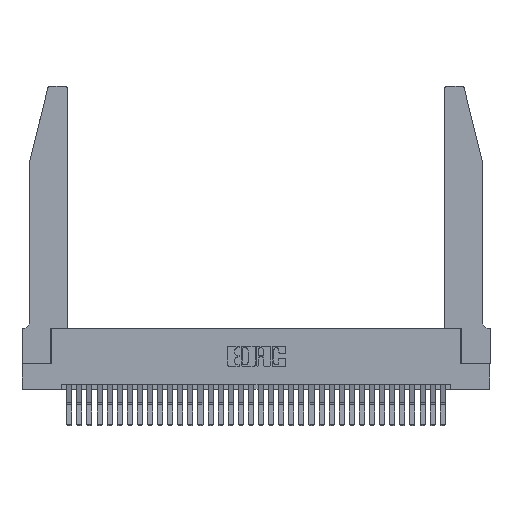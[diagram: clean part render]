
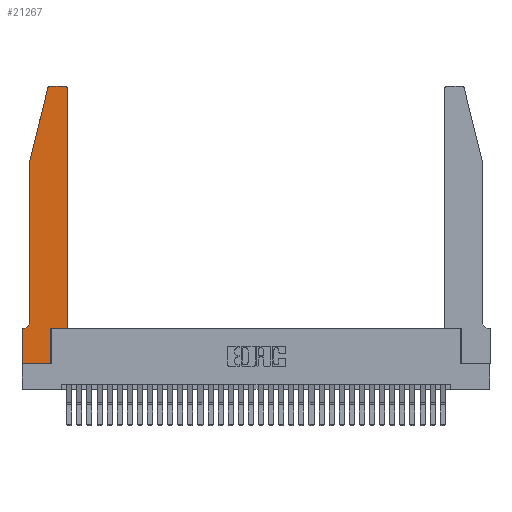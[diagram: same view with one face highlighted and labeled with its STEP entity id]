
A CAD part, top view. The second image highlights one B-rep face of the part: STEP entity #21267.
In plain terms, the highlighted planar face has unit normal (0, 0, 1).
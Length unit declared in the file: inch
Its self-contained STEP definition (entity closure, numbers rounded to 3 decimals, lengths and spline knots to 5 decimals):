
#935 = DIRECTION ( 'NONE',  ( 0., -1., 0. ) ) ;
#1201 = ORIENTED_EDGE ( 'NONE', *, *, #31372, .T. ) ;
#1291 = CARTESIAN_POINT ( 'NONE',  ( 0.0755, 2., 0.37 ) ) ;
#1376 = ORIENTED_EDGE ( 'NONE', *, *, #2684, .T. ) ;
#1956 = DIRECTION ( 'NONE',  ( 1., 0., 0. ) ) ;
#2573 = LINE ( 'NONE', #11858, #15707 ) ;
#2684 = EDGE_CURVE ( 'NONE', #17041, #10443, #32523, .T. ) ;
#2877 = CARTESIAN_POINT ( 'NONE',  ( 0., 0., 0.37 ) ) ;
#3199 = VECTOR ( 'NONE', #15643, 39.37008 ) ;
#3333 = LINE ( 'NONE', #8171, #29338 ) ;
#3379 = CARTESIAN_POINT ( 'NONE',  ( 0.0755, 0.35, 0.37 ) ) ;
#3596 = LINE ( 'NONE', #31079, #3199 ) ;
#3832 = ORIENTED_EDGE ( 'NONE', *, *, #15936, .T. ) ;
#4374 = DIRECTION ( 'NONE',  ( 0., 1., 0. ) ) ;
#4702 = CARTESIAN_POINT ( 'NONE',  ( 0.2865, 0.35, 0.37 ) ) ;
#5097 = VERTEX_POINT ( 'NONE', #31249 ) ;
#5255 = CARTESIAN_POINT ( 'NONE',  ( 0.0755, 2., 0.37 ) ) ;
#5286 = DIRECTION ( 'NONE',  ( 1., 0., 0. ) ) ;
#6070 = ORIENTED_EDGE ( 'NONE', *, *, #16744, .T. ) ;
#6346 = VERTEX_POINT ( 'NONE', #7007 ) ;
#6767 = EDGE_CURVE ( 'NONE', #12566, #17512, #3596, .T. ) ;
#7007 = CARTESIAN_POINT ( 'NONE',  ( 0.4505, 2.72, 0.37 ) ) ;
#7131 = AXIS2_PLACEMENT_3D ( 'NONE', #7559, #13362, #5286 ) ;
#7261 = AXIS2_PLACEMENT_3D ( 'NONE', #22783, #31485, #20400 ) ;
#7324 = PLANE ( 'NONE',  #7261 ) ;
#7491 = FACE_OUTER_BOUND ( 'NONE', #23174, .T. ) ;
#7559 = CARTESIAN_POINT ( 'NONE',  ( 0.4205, 2.72, 0.37 ) ) ;
#7577 = LINE ( 'NONE', #17139, #25419 ) ;
#7645 = CARTESIAN_POINT ( 'NONE',  ( 0.284, 2.72, 0.37 ) ) ;
#7892 = ORIENTED_EDGE ( 'NONE', *, *, #26715, .T. ) ;
#8171 = CARTESIAN_POINT ( 'NONE',  ( 0., 0., 0.37 ) ) ;
#8234 = CARTESIAN_POINT ( 'NONE',  ( 0., 0., 0.37 ) ) ;
#8263 = CARTESIAN_POINT ( 'NONE',  ( 0.0755, 0.42, 0.37 ) ) ;
#8727 = DIRECTION ( 'NONE',  ( -1., 0., 0. ) ) ;
#10402 = VERTEX_POINT ( 'NONE', #13631 ) ;
#10443 = VERTEX_POINT ( 'NONE', #13195 ) ;
#11034 = AXIS2_PLACEMENT_3D ( 'NONE', #7645, #15710, #1956 ) ;
#11858 = CARTESIAN_POINT ( 'NONE',  ( 0.2865, 0.35, 0.37 ) ) ;
#12290 = LINE ( 'NONE', #20895, #33139 ) ;
#12566 = VERTEX_POINT ( 'NONE', #4702 ) ;
#13195 = CARTESIAN_POINT ( 'NONE',  ( 0.25487, 2.72718, 0.37 ) ) ;
#13362 = DIRECTION ( 'NONE',  ( 0., 0., 1. ) ) ;
#13631 = CARTESIAN_POINT ( 'NONE',  ( 0., 0.35, 0.37 ) ) ;
#13691 = LINE ( 'NONE', #18768, #25615 ) ;
#15182 = VERTEX_POINT ( 'NONE', #8263 ) ;
#15643 = DIRECTION ( 'NONE',  ( 1., 0., 0. ) ) ;
#15707 = VECTOR ( 'NONE', #33638, 39.37008 ) ;
#15710 = DIRECTION ( 'NONE',  ( 0., 0., 1. ) ) ;
#15936 = EDGE_CURVE ( 'NONE', #20527, #12566, #2573, .T. ) ;
#16136 = CARTESIAN_POINT ( 'NONE',  ( 0.2865, 0., 0.37 ) ) ;
#16158 = DIRECTION ( 'NONE',  ( -1., 0., 0. ) ) ;
#16230 = EDGE_CURVE ( 'NONE', #21642, #20527, #3333, .T. ) ;
#16500 = DIRECTION ( 'NONE',  ( 0., -1., 0. ) ) ;
#16620 = LINE ( 'NONE', #3379, #26093 ) ;
#16744 = EDGE_CURVE ( 'NONE', #10402, #21642, #32258, .T. ) ;
#16777 = DIRECTION ( 'NONE',  ( -1., 0., 0. ) ) ;
#16816 = EDGE_CURVE ( 'NONE', #17512, #6346, #7577, .T. ) ;
#16993 = DIRECTION ( 'NONE',  ( 0., 0., -1. ) ) ;
#17041 = VERTEX_POINT ( 'NONE', #19272 ) ;
#17139 = CARTESIAN_POINT ( 'NONE',  ( 0.4505, 0.35, 0.37 ) ) ;
#17512 = VERTEX_POINT ( 'NONE', #26223 ) ;
#18211 = ORIENTED_EDGE ( 'NONE', *, *, #24803, .T. ) ;
#18369 = ORIENTED_EDGE ( 'NONE', *, *, #25897, .T. ) ;
#18768 = CARTESIAN_POINT ( 'NONE',  ( 0.2605, 2.75, 0.37 ) ) ;
#19272 = CARTESIAN_POINT ( 'NONE',  ( 0.284, 2.75, 0.37 ) ) ;
#19880 = CIRCLE ( 'NONE', #7131, 0.03 ) ;
#20400 = DIRECTION ( 'NONE',  ( 1., 0., 0. ) ) ;
#20527 = VERTEX_POINT ( 'NONE', #16136 ) ;
#20772 = DIRECTION ( 'NONE',  ( -0.239, -0.971, 0. ) ) ;
#20799 = ORIENTED_EDGE ( 'NONE', *, *, #16230, .T. ) ;
#20895 = CARTESIAN_POINT ( 'NONE',  ( 0.0755, 2., 0.37 ) ) ;
#21267 = ADVANCED_FACE ( 'NONE', ( #7491 ), #7324, .T. ) ;
#21642 = VERTEX_POINT ( 'NONE', #2877 ) ;
#22783 = CARTESIAN_POINT ( 'NONE',  ( 0., 0.35, 0.37 ) ) ;
#22897 = ORIENTED_EDGE ( 'NONE', *, *, #28335, .T. ) ;
#22963 = VERTEX_POINT ( 'NONE', #29801 ) ;
#23174 = EDGE_LOOP ( 'NONE', ( #18369, #1376, #22897, #1201, #18211, #7892, #6070, #20799, #3832, #27539, #25105, #32581 ) ) ;
#24052 = CIRCLE ( 'NONE', #26713, 0.07 ) ;
#24074 = LINE ( 'NONE', #1291, #29592 ) ;
#24482 = DIRECTION ( 'NONE',  ( 1., 0., 0. ) ) ;
#24803 = EDGE_CURVE ( 'NONE', #15182, #5097, #24052, .T. ) ;
#25013 = VECTOR ( 'NONE', #16500, 39.37008 ) ;
#25105 = ORIENTED_EDGE ( 'NONE', *, *, #16816, .T. ) ;
#25419 = VECTOR ( 'NONE', #4374, 39.37008 ) ;
#25615 = VECTOR ( 'NONE', #16158, 39.37008 ) ;
#25897 = EDGE_CURVE ( 'NONE', #22963, #17041, #13691, .T. ) ;
#26093 = VECTOR ( 'NONE', #16777, 39.37008 ) ;
#26223 = CARTESIAN_POINT ( 'NONE',  ( 0.4505, 0.35, 0.37 ) ) ;
#26713 = AXIS2_PLACEMENT_3D ( 'NONE', #27387, #16993, #8727 ) ;
#26715 = EDGE_CURVE ( 'NONE', #5097, #10402, #16620, .T. ) ;
#27387 = CARTESIAN_POINT ( 'NONE',  ( 0.0055, 0.42, 0.37 ) ) ;
#27539 = ORIENTED_EDGE ( 'NONE', *, *, #6767, .T. ) ;
#27979 = VERTEX_POINT ( 'NONE', #5255 ) ;
#28335 = EDGE_CURVE ( 'NONE', #10443, #27979, #12290, .T. ) ;
#29243 = EDGE_CURVE ( 'NONE', #6346, #22963, #19880, .T. ) ;
#29338 = VECTOR ( 'NONE', #24482, 39.37008 ) ;
#29592 = VECTOR ( 'NONE', #935, 39.37008 ) ;
#29801 = CARTESIAN_POINT ( 'NONE',  ( 0.4205, 2.75, 0.37 ) ) ;
#31079 = CARTESIAN_POINT ( 'NONE',  ( 0.4505, 0.35, 0.37 ) ) ;
#31249 = CARTESIAN_POINT ( 'NONE',  ( 0.0055, 0.35, 0.37 ) ) ;
#31372 = EDGE_CURVE ( 'NONE', #27979, #15182, #24074, .T. ) ;
#31485 = DIRECTION ( 'NONE',  ( 0., 0., 1. ) ) ;
#32258 = LINE ( 'NONE', #8234, #25013 ) ;
#32523 = CIRCLE ( 'NONE', #11034, 0.03 ) ;
#32581 = ORIENTED_EDGE ( 'NONE', *, *, #29243, .T. ) ;
#33139 = VECTOR ( 'NONE', #20772, 39.37008 ) ;
#33638 = DIRECTION ( 'NONE',  ( 0., 1., 0. ) ) ;
